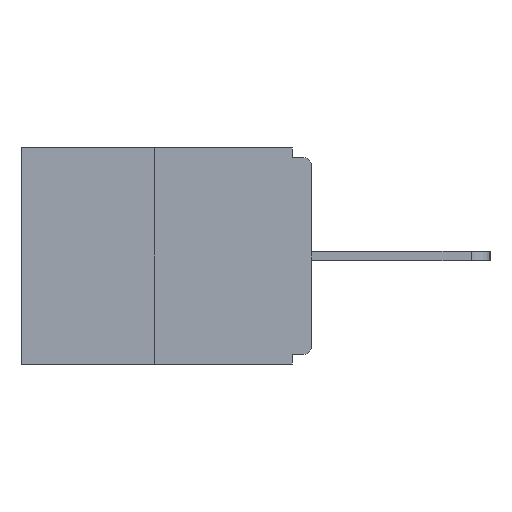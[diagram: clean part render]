
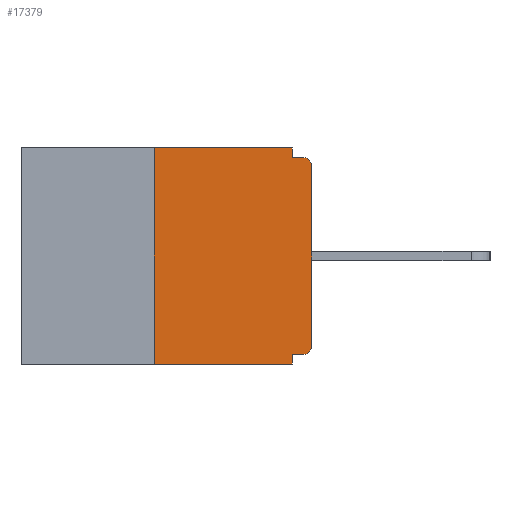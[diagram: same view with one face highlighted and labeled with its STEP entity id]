
A CAD part, left-side view. The second image highlights one B-rep face of the part: STEP entity #17379.
In plain terms, the highlighted planar face has unit normal (-1, 0, 0).
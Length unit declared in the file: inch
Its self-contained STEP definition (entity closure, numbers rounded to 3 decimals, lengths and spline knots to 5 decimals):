
#79 = VECTOR ( 'NONE', #21953, 39.37008 ) ;
#84 = CARTESIAN_POINT ( 'NONE',  ( 0., 0., -0.328 ) ) ;
#481 = VERTEX_POINT ( 'NONE', #2250 ) ;
#564 = EDGE_CURVE ( 'NONE', #25092, #9564, #5747, .T. ) ;
#724 = VERTEX_POINT ( 'NONE', #25512 ) ;
#953 = AXIS2_PLACEMENT_3D ( 'NONE', #22834, #25016, #10325 ) ;
#1819 = CIRCLE ( 'NONE', #953, 0.015 ) ;
#1974 = ORIENTED_EDGE ( 'NONE', *, *, #14733, .T. ) ;
#2142 = VERTEX_POINT ( 'NONE', #9635 ) ;
#2250 = CARTESIAN_POINT ( 'NONE',  ( 0., 0.031, -0.328 ) ) ;
#2328 = VECTOR ( 'NONE', #7655, 39.37008 ) ;
#3260 = DIRECTION ( 'NONE',  ( 0., 0., -1. ) ) ;
#3348 = ORIENTED_EDGE ( 'NONE', *, *, #7746, .T. ) ;
#3436 = DIRECTION ( 'NONE',  ( 1., 0., 0. ) ) ;
#3576 = DIRECTION ( 'NONE',  ( 0., 0., -1. ) ) ;
#3927 = EDGE_LOOP ( 'NONE', ( #26374, #7170, #12453, #21023, #12179, #1974, #3348, #5496, #8313, #22167 ) ) ;
#4126 = VECTOR ( 'NONE', #20522, 39.37008 ) ;
#4401 = DIRECTION ( 'NONE',  ( 0., -1., 0. ) ) ;
#4485 = CARTESIAN_POINT ( 'NONE',  ( 0., 0.031, -0.343 ) ) ;
#5373 = FACE_OUTER_BOUND ( 'NONE', #3927, .T. ) ;
#5496 = ORIENTED_EDGE ( 'NONE', *, *, #14816, .T. ) ;
#5747 = LINE ( 'NONE', #20454, #2328 ) ;
#5825 = LINE ( 'NONE', #24612, #4126 ) ;
#5979 = DIRECTION ( 'NONE',  ( 0., 1., 0. ) ) ;
#7085 = EDGE_CURVE ( 'NONE', #24992, #25092, #24288, .T. ) ;
#7170 = ORIENTED_EDGE ( 'NONE', *, *, #25918, .F. ) ;
#7256 = VECTOR ( 'NONE', #3576, 39.37008 ) ;
#7526 = CARTESIAN_POINT ( 'NONE',  ( 0., 0.46, 0. ) ) ;
#7655 = DIRECTION ( 'NONE',  ( 0., -1., 0. ) ) ;
#7671 = CARTESIAN_POINT ( 'NONE',  ( 0., 0.031, 0. ) ) ;
#7746 = EDGE_CURVE ( 'NONE', #13892, #17420, #17553, .T. ) ;
#8223 = CARTESIAN_POINT ( 'NONE',  ( 0., 0.46, -0.343 ) ) ;
#8313 = ORIENTED_EDGE ( 'NONE', *, *, #564, .F. ) ;
#8425 = DIRECTION ( 'NONE',  ( 0., -1., 0. ) ) ;
#8777 = VECTOR ( 'NONE', #5979, 39.37008 ) ;
#8953 = EDGE_CURVE ( 'NONE', #481, #22607, #5825, .T. ) ;
#9249 = DIRECTION ( 'NONE',  ( 0., 0., 1. ) ) ;
#9564 = VERTEX_POINT ( 'NONE', #16808 ) ;
#9635 = CARTESIAN_POINT ( 'NONE',  ( 0., 0.25, -0.343 ) ) ;
#9933 = DIRECTION ( 'NONE',  ( -1., 0., 0. ) ) ;
#10325 = DIRECTION ( 'NONE',  ( 0., 0., -1. ) ) ;
#11018 = EDGE_CURVE ( 'NONE', #2142, #22607, #22785, .T. ) ;
#11366 = CIRCLE ( 'NONE', #19175, 0.015 ) ;
#11548 = VECTOR ( 'NONE', #8425, 39.37008 ) ;
#12179 = ORIENTED_EDGE ( 'NONE', *, *, #14887, .F. ) ;
#12210 = LINE ( 'NONE', #84, #8777 ) ;
#12215 = CARTESIAN_POINT ( 'NONE',  ( 0., 0.46, 0. ) ) ;
#12453 = ORIENTED_EDGE ( 'NONE', *, *, #11018, .T. ) ;
#13892 = VERTEX_POINT ( 'NONE', #14490 ) ;
#14490 = CARTESIAN_POINT ( 'NONE',  ( 0., 0., -0.313 ) ) ;
#14733 = EDGE_CURVE ( 'NONE', #724, #13892, #11366, .T. ) ;
#14816 = EDGE_CURVE ( 'NONE', #17420, #9564, #1819, .T. ) ;
#14887 = EDGE_CURVE ( 'NONE', #724, #481, #12210, .T. ) ;
#16808 = CARTESIAN_POINT ( 'NONE',  ( 0., 0.015, -0.015 ) ) ;
#16813 = VECTOR ( 'NONE', #4401, 39.37008 ) ;
#17379 = ADVANCED_FACE ( 'NONE', ( #5373 ), #26152, .F. ) ;
#17420 = VERTEX_POINT ( 'NONE', #20046 ) ;
#17553 = LINE ( 'NONE', #23941, #19438 ) ;
#18763 = LINE ( 'NONE', #12215, #11548 ) ;
#19175 = AXIS2_PLACEMENT_3D ( 'NONE', #24496, #9933, #3260 ) ;
#19438 = VECTOR ( 'NONE', #9249, 39.37008 ) ;
#19699 = CARTESIAN_POINT ( 'NONE',  ( 0., 0.031, 0. ) ) ;
#19779 = CARTESIAN_POINT ( 'NONE',  ( 0., 0.25, 0. ) ) ;
#20041 = LINE ( 'NONE', #26013, #79 ) ;
#20046 = CARTESIAN_POINT ( 'NONE',  ( 0., 0., -0.03 ) ) ;
#20454 = CARTESIAN_POINT ( 'NONE',  ( 0., 0., -0.015 ) ) ;
#20522 = DIRECTION ( 'NONE',  ( 0., 0., -1. ) ) ;
#21023 = ORIENTED_EDGE ( 'NONE', *, *, #8953, .F. ) ;
#21953 = DIRECTION ( 'NONE',  ( 0., 0., 1. ) ) ;
#21958 = DIRECTION ( 'NONE',  ( 0., 0., -1. ) ) ;
#22167 = ORIENTED_EDGE ( 'NONE', *, *, #7085, .F. ) ;
#22607 = VERTEX_POINT ( 'NONE', #4485 ) ;
#22785 = LINE ( 'NONE', #8223, #16813 ) ;
#22834 = CARTESIAN_POINT ( 'NONE',  ( 0., 0.015, -0.03 ) ) ;
#23941 = CARTESIAN_POINT ( 'NONE',  ( 0., 0., 0. ) ) ;
#24288 = LINE ( 'NONE', #7671, #7256 ) ;
#24496 = CARTESIAN_POINT ( 'NONE',  ( 0., 0.015, -0.313 ) ) ;
#24612 = CARTESIAN_POINT ( 'NONE',  ( 0., 0.031, -0.343 ) ) ;
#24881 = EDGE_CURVE ( 'NONE', #26009, #24992, #18763, .T. ) ;
#24992 = VERTEX_POINT ( 'NONE', #19699 ) ;
#25016 = DIRECTION ( 'NONE',  ( -1., 0., 0. ) ) ;
#25092 = VERTEX_POINT ( 'NONE', #26215 ) ;
#25314 = AXIS2_PLACEMENT_3D ( 'NONE', #7526, #3436, #21958 ) ;
#25512 = CARTESIAN_POINT ( 'NONE',  ( 0., 0.015, -0.328 ) ) ;
#25918 = EDGE_CURVE ( 'NONE', #2142, #26009, #20041, .T. ) ;
#26009 = VERTEX_POINT ( 'NONE', #19779 ) ;
#26013 = CARTESIAN_POINT ( 'NONE',  ( 0., 0.25, 0. ) ) ;
#26152 = PLANE ( 'NONE',  #25314 ) ;
#26215 = CARTESIAN_POINT ( 'NONE',  ( 0., 0.031, -0.015 ) ) ;
#26374 = ORIENTED_EDGE ( 'NONE', *, *, #24881, .F. ) ;
